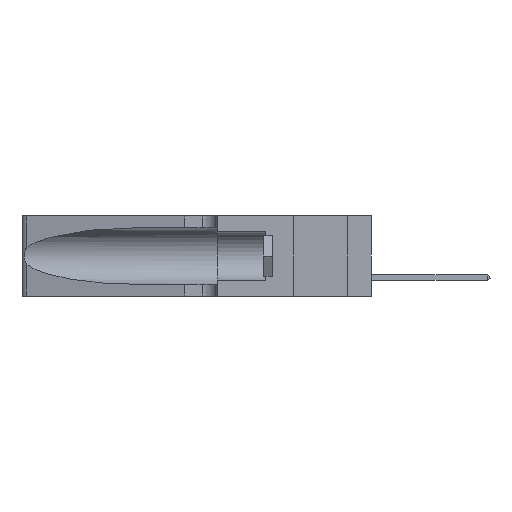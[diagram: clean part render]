
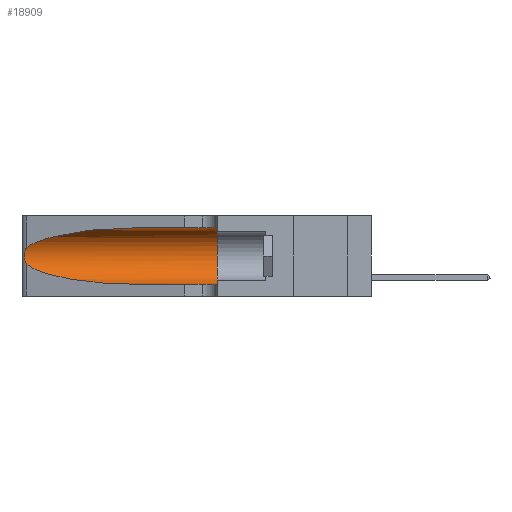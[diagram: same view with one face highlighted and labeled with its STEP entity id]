
A CAD part, left-side view. The second image highlights one B-rep face of the part: STEP entity #18909.
In plain terms, the highlighted cylindrical face has radius 3.308 mm (diameter 6.617 mm), a partial arc.
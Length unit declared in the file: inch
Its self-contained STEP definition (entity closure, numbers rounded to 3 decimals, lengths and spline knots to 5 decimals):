
#386 = CARTESIAN_POINT ( 'NONE',  ( 0.1305, 0.35, 0.05475 ) ) ;
#463 = AXIS2_PLACEMENT_3D ( 'NONE', #15462, #13110, #2670 ) ;
#822 =( BOUNDED_CURVE ( )  B_SPLINE_CURVE ( 3, ( #23869, #19312, #15000, #4594 ),
 .UNSPECIFIED., .F., .T. ) 
 B_SPLINE_CURVE_WITH_KNOTS ( ( 4, 4 ),
 ( 3.44316, 4.71239 ),
 .UNSPECIFIED. ) 
 CURVE ( )  GEOMETRIC_REPRESENTATION_ITEM ( )  RATIONAL_B_SPLINE_CURVE ( ( 1., 0.87, 0.87, 1. ) ) 
 REPRESENTATION_ITEM ( '' )  );
#851 = EDGE_CURVE ( 'NONE', #8381, #7160, #21515, .T. ) ;
#1103 = CIRCLE ( 'NONE', #9997, 0.13025 ) ;
#1175 = CARTESIAN_POINT ( 'NONE',  ( 0.26018, 1.23835, 0.19895 ) ) ;
#1458 = CARTESIAN_POINT ( 'NONE',  ( 0.26017, 1.23833, 0.17102 ) ) ;
#1619 = CARTESIAN_POINT ( 'NONE',  ( 0.18966, 0.96281, 0.31525 ) ) ;
#1866 = CARTESIAN_POINT ( 'NONE',  ( 0.25487, 1.22718, 0.14631 ) ) ;
#2602 = DIRECTION ( 'NONE',  ( 0., -1., 0. ) ) ;
#2670 = DIRECTION ( 'NONE',  ( 0., 0., -1. ) ) ;
#2683 = VERTEX_POINT ( 'NONE', #17076 ) ;
#3737 = CARTESIAN_POINT ( 'NONE',  ( 0.25487, 1.22718, 0.22369 ) ) ;
#4421 = VERTEX_POINT ( 'NONE', #26667 ) ;
#4594 = CARTESIAN_POINT ( 'NONE',  ( 0.1305, 0.72297, 0.05475 ) ) ;
#4998 = CARTESIAN_POINT ( 'NONE',  ( 0.1305, 1.61858, 0.31525 ) ) ;
#5905 = CARTESIAN_POINT ( 'NONE',  ( 0.25856, 1.23593, 0.16098 ) ) ;
#6031 = ORIENTED_EDGE ( 'NONE', *, *, #851, .T. ) ;
#6164 = EDGE_CURVE ( 'NONE', #4421, #7160, #1103, .T. ) ;
#7160 = VERTEX_POINT ( 'NONE', #386 ) ;
#7978 = CARTESIAN_POINT ( 'NONE',  ( 0.1305, 0.72297, 0.05475 ) ) ;
#8040 = CARTESIAN_POINT ( 'NONE',  ( 0.1305, 0.72297, 0.31525 ) ) ;
#8049 = CARTESIAN_POINT ( 'NONE',  ( 0.25789, 1.23486, 0.15765 ) ) ;
#8381 = VERTEX_POINT ( 'NONE', #7978 ) ;
#8535 = VERTEX_POINT ( 'NONE', #3737 ) ;
#8604 = ORIENTED_EDGE ( 'NONE', *, *, #19587, .F. ) ;
#9245 = VECTOR ( 'NONE', #2602, 39.37008 ) ;
#9997 = AXIS2_PLACEMENT_3D ( 'NONE', #16913, #18486, #19253 ) ;
#10019 = CARTESIAN_POINT ( 'NONE',  ( 0.25555, 1.22994, 0.2215 ) ) ;
#10214 = CARTESIAN_POINT ( 'NONE',  ( 0.26075, 1.23896, 0.19203 ) ) ;
#12019 = FACE_OUTER_BOUND ( 'NONE', #17280, .T. ) ;
#12245 = LINE ( 'NONE', #4998, #9245 ) ;
#12254 = CARTESIAN_POINT ( 'NONE',  ( 0.26075, 1.23896, 0.178 ) ) ;
#13110 = DIRECTION ( 'NONE',  ( 0., -1., 0. ) ) ;
#13377 = EDGE_CURVE ( 'NONE', #8535, #14416, #20280, .T. ) ;
#14416 = VERTEX_POINT ( 'NONE', #1866 ) ;
#15000 = CARTESIAN_POINT ( 'NONE',  ( 0.18966, 0.96281, 0.05475 ) ) ;
#15462 = CARTESIAN_POINT ( 'NONE',  ( 0.1305, 1.61858, 0.185 ) ) ;
#15563 = ORIENTED_EDGE ( 'NONE', *, *, #6164, .F. ) ;
#16217 = CARTESIAN_POINT ( 'NONE',  ( 0.25487, 1.22718, 0.14631 ) ) ;
#16302 = CARTESIAN_POINT ( 'NONE',  ( 0.25487, 1.22718, 0.22369 ) ) ;
#16477 = VECTOR ( 'NONE', #21644, 39.37008 ) ;
#16658 = CARTESIAN_POINT ( 'NONE',  ( 0.25487, 1.22718, 0.22369 ) ) ;
#16913 = CARTESIAN_POINT ( 'NONE',  ( 0.1305, 0.35, 0.185 ) ) ;
#17069 = ORIENTED_EDGE ( 'NONE', *, *, #26935, .T. ) ;
#17076 = CARTESIAN_POINT ( 'NONE',  ( 0.1305, 0.72297, 0.31525 ) ) ;
#17280 = EDGE_LOOP ( 'NONE', ( #17069, #20287, #23145, #6031, #15563, #8604 ) ) ;
#17700 = CYLINDRICAL_SURFACE ( 'NONE', #463, 0.13025 ) ;
#17719 = EDGE_CURVE ( 'NONE', #14416, #8381, #822, .T. ) ;
#17841 =( BOUNDED_CURVE ( )  B_SPLINE_CURVE ( 3, ( #8040, #1619, #23030, #16658 ),
 .UNSPECIFIED., .F., .F. ) 
 B_SPLINE_CURVE_WITH_KNOTS ( ( 4, 4 ),
 ( 1.5708, 2.84003 ),
 .UNSPECIFIED. ) 
 CURVE ( )  GEOMETRIC_REPRESENTATION_ITEM ( )  RATIONAL_B_SPLINE_CURVE ( ( 1., 0.87, 0.87, 1. ) ) 
 REPRESENTATION_ITEM ( '' )  );
#18486 = DIRECTION ( 'NONE',  ( 0., 1., 0. ) ) ;
#18712 = CARTESIAN_POINT ( 'NONE',  ( 0.25787, 1.23484, 0.2124 ) ) ;
#18909 = ADVANCED_FACE ( 'NONE', ( #12019 ), #17700, .F. ) ;
#19253 = DIRECTION ( 'NONE',  ( 0., 0., 1. ) ) ;
#19312 = CARTESIAN_POINT ( 'NONE',  ( 0.2373, 1.15595, 0.08982 ) ) ;
#19575 = CARTESIAN_POINT ( 'NONE',  ( 0.1305, 1.61858, 0.05475 ) ) ;
#19587 = EDGE_CURVE ( 'NONE', #2683, #4421, #12245, .T. ) ;
#20280 = B_SPLINE_CURVE_WITH_KNOTS ( 'NONE', 3,
 ( #16302, #10019, #24958, #18712, #27118, #1175, #10214, #12254, #1458, #5905, #8049, #27217, #23036, #16217 ),
 .UNSPECIFIED., .F., .F.,
 ( 4, 2, 2, 2, 2, 2, 4 ),
 ( 0., 0.00027, 0.00053, 0.00107, 0.0016, 0.00187, 0.00214 ),
 .UNSPECIFIED. ) ;
#20287 = ORIENTED_EDGE ( 'NONE', *, *, #13377, .T. ) ;
#21515 = LINE ( 'NONE', #19575, #16477 ) ;
#21644 = DIRECTION ( 'NONE',  ( 0., -1., 0. ) ) ;
#23030 = CARTESIAN_POINT ( 'NONE',  ( 0.2373, 1.15595, 0.28018 ) ) ;
#23036 = CARTESIAN_POINT ( 'NONE',  ( 0.25555, 1.22993, 0.14849 ) ) ;
#23145 = ORIENTED_EDGE ( 'NONE', *, *, #17719, .T. ) ;
#23869 = CARTESIAN_POINT ( 'NONE',  ( 0.25487, 1.22718, 0.14631 ) ) ;
#24958 = CARTESIAN_POINT ( 'NONE',  ( 0.25639, 1.23184, 0.21858 ) ) ;
#26667 = CARTESIAN_POINT ( 'NONE',  ( 0.1305, 0.35, 0.31525 ) ) ;
#26935 = EDGE_CURVE ( 'NONE', #2683, #8535, #17841, .T. ) ;
#27118 = CARTESIAN_POINT ( 'NONE',  ( 0.25854, 1.2359, 0.20912 ) ) ;
#27217 = CARTESIAN_POINT ( 'NONE',  ( 0.25639, 1.23186, 0.15144 ) ) ;
